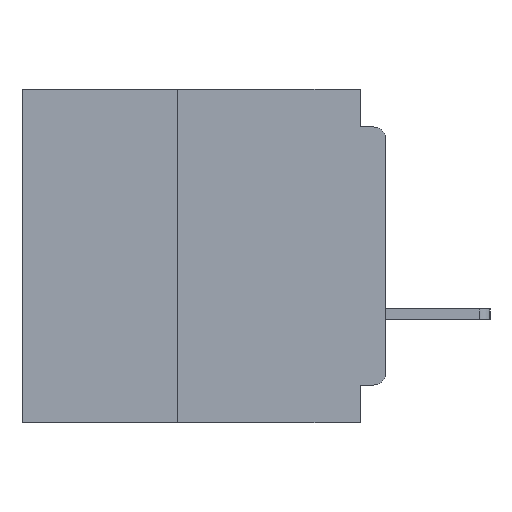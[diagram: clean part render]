
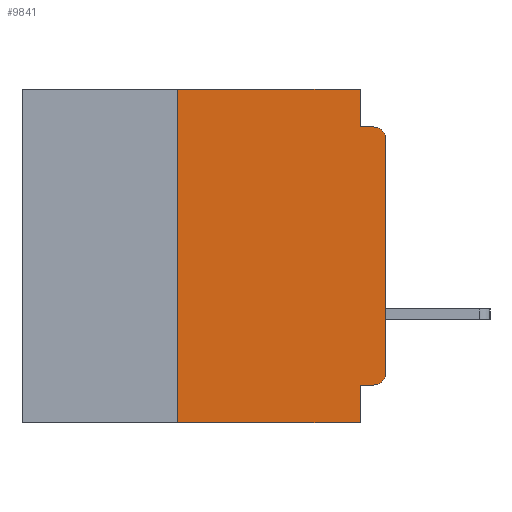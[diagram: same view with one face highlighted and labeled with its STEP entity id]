
A CAD part, left-side view. The second image highlights one B-rep face of the part: STEP entity #9841.
In plain terms, the highlighted planar face has unit normal (-1, 0, 0).
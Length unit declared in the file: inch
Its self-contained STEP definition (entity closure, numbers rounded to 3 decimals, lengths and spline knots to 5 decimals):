
#498 = DIRECTION ( 'NONE',  ( 0., 0., -1. ) ) ;
#1784 = ORIENTED_EDGE ( 'NONE', *, *, #11485, .F. ) ;
#2168 = VECTOR ( 'NONE', #498, 39.37008 ) ;
#2342 = CARTESIAN_POINT ( 'NONE',  ( 0., 0.015, -0.34 ) ) ;
#2679 = CARTESIAN_POINT ( 'NONE',  ( 0., 0.031, 0. ) ) ;
#3452 = DIRECTION ( 'NONE',  ( 0., 0., -1. ) ) ;
#3649 = VECTOR ( 'NONE', #39063, 39.37008 ) ;
#3735 = ORIENTED_EDGE ( 'NONE', *, *, #31207, .T. ) ;
#4716 = DIRECTION ( 'NONE',  ( 0., 1., 0. ) ) ;
#5376 = DIRECTION ( 'NONE',  ( 0., 0., -1. ) ) ;
#5522 = CARTESIAN_POINT ( 'NONE',  ( 0., 0.437, 0. ) ) ;
#5532 = ORIENTED_EDGE ( 'NONE', *, *, #30784, .F. ) ;
#6460 = CARTESIAN_POINT ( 'NONE',  ( 0., 0.015, -0.06 ) ) ;
#6625 = AXIS2_PLACEMENT_3D ( 'NONE', #36912, #30964, #12550 ) ;
#7066 = LINE ( 'NONE', #27614, #14084 ) ;
#7103 = VECTOR ( 'NONE', #31562, 39.37008 ) ;
#7303 = VERTEX_POINT ( 'NONE', #2679 ) ;
#7372 = EDGE_CURVE ( 'NONE', #10352, #23011, #22905, .T. ) ;
#8560 = CARTESIAN_POINT ( 'NONE',  ( 0., 0.25, -0.4 ) ) ;
#8852 = VECTOR ( 'NONE', #4716, 39.37008 ) ;
#9121 = CARTESIAN_POINT ( 'NONE',  ( 0., 0.015, -0.355 ) ) ;
#9322 = AXIS2_PLACEMENT_3D ( 'NONE', #6460, #27766, #9464 ) ;
#9464 = DIRECTION ( 'NONE',  ( 0., 0., -1. ) ) ;
#9841 = ADVANCED_FACE ( 'NONE', ( #22659 ), #27706, .F. ) ;
#9963 = EDGE_CURVE ( 'NONE', #17622, #19025, #16891, .T. ) ;
#10143 = CARTESIAN_POINT ( 'NONE',  ( 0., 0., -0.045 ) ) ;
#10352 = VERTEX_POINT ( 'NONE', #30657 ) ;
#10686 = LINE ( 'NONE', #5522, #3649 ) ;
#11402 = VECTOR ( 'NONE', #35958, 39.37008 ) ;
#11476 = CARTESIAN_POINT ( 'NONE',  ( 0., 0., 0. ) ) ;
#11485 = EDGE_CURVE ( 'NONE', #21725, #7303, #10686, .T. ) ;
#12081 = ORIENTED_EDGE ( 'NONE', *, *, #13093, .T. ) ;
#12195 = DIRECTION ( 'NONE',  ( 0., -1., 0. ) ) ;
#12343 = CARTESIAN_POINT ( 'NONE',  ( 0., 0.031, -0.4 ) ) ;
#12550 = DIRECTION ( 'NONE',  ( 0., 0., -1. ) ) ;
#13093 = EDGE_CURVE ( 'NONE', #17622, #28622, #23886, .T. ) ;
#14084 = VECTOR ( 'NONE', #12195, 39.37008 ) ;
#16891 = LINE ( 'NONE', #32132, #8852 ) ;
#17622 = VERTEX_POINT ( 'NONE', #9121 ) ;
#18445 = ORIENTED_EDGE ( 'NONE', *, *, #36639, .T. ) ;
#18554 = CARTESIAN_POINT ( 'NONE',  ( 0., 0.031, 0. ) ) ;
#19025 = VERTEX_POINT ( 'NONE', #19758 ) ;
#19479 = LINE ( 'NONE', #11476, #11402 ) ;
#19758 = CARTESIAN_POINT ( 'NONE',  ( 0., 0.031, -0.355 ) ) ;
#21395 = EDGE_CURVE ( 'NONE', #23508, #21725, #31826, .T. ) ;
#21725 = VERTEX_POINT ( 'NONE', #36845 ) ;
#22067 = ORIENTED_EDGE ( 'NONE', *, *, #24226, .F. ) ;
#22079 = ORIENTED_EDGE ( 'NONE', *, *, #9963, .F. ) ;
#22505 = AXIS2_PLACEMENT_3D ( 'NONE', #2342, #23511, #5376 ) ;
#22659 = FACE_OUTER_BOUND ( 'NONE', #28017, .T. ) ;
#22905 = CIRCLE ( 'NONE', #9322, 0.015 ) ;
#23011 = VERTEX_POINT ( 'NONE', #33696 ) ;
#23231 = VERTEX_POINT ( 'NONE', #28603 ) ;
#23508 = VERTEX_POINT ( 'NONE', #8560 ) ;
#23511 = DIRECTION ( 'NONE',  ( -1., 0., 0. ) ) ;
#23631 = VECTOR ( 'NONE', #35015, 39.37008 ) ;
#23686 = EDGE_CURVE ( 'NONE', #19025, #23231, #26373, .T. ) ;
#23886 = CIRCLE ( 'NONE', #22505, 0.015 ) ;
#24226 = EDGE_CURVE ( 'NONE', #7303, #28901, #35487, .T. ) ;
#25388 = VECTOR ( 'NONE', #3452, 39.37008 ) ;
#25873 = ORIENTED_EDGE ( 'NONE', *, *, #23686, .F. ) ;
#26373 = LINE ( 'NONE', #12343, #25388 ) ;
#27614 = CARTESIAN_POINT ( 'NONE',  ( 0., 0.437, -0.4 ) ) ;
#27706 = PLANE ( 'NONE',  #6625 ) ;
#27766 = DIRECTION ( 'NONE',  ( -1., 0., 0. ) ) ;
#28017 = EDGE_LOOP ( 'NONE', ( #18445, #36477, #5532, #22067, #1784, #31805, #3735, #25873, #22079, #12081 ) ) ;
#28572 = CARTESIAN_POINT ( 'NONE',  ( 0., 0.031, -0.045 ) ) ;
#28603 = CARTESIAN_POINT ( 'NONE',  ( 0., 0.031, -0.4 ) ) ;
#28622 = VERTEX_POINT ( 'NONE', #33280 ) ;
#28901 = VERTEX_POINT ( 'NONE', #28572 ) ;
#30657 = CARTESIAN_POINT ( 'NONE',  ( 0., 0., -0.06 ) ) ;
#30784 = EDGE_CURVE ( 'NONE', #28901, #23011, #31473, .T. ) ;
#30964 = DIRECTION ( 'NONE',  ( 1., 0., 0. ) ) ;
#31207 = EDGE_CURVE ( 'NONE', #23508, #23231, #7066, .T. ) ;
#31473 = LINE ( 'NONE', #10143, #7103 ) ;
#31562 = DIRECTION ( 'NONE',  ( 0., -1., 0. ) ) ;
#31805 = ORIENTED_EDGE ( 'NONE', *, *, #21395, .F. ) ;
#31826 = LINE ( 'NONE', #31960, #23631 ) ;
#31960 = CARTESIAN_POINT ( 'NONE',  ( 0., 0.25, -0.4 ) ) ;
#32132 = CARTESIAN_POINT ( 'NONE',  ( 0., 0., -0.355 ) ) ;
#33280 = CARTESIAN_POINT ( 'NONE',  ( 0., 0., -0.34 ) ) ;
#33696 = CARTESIAN_POINT ( 'NONE',  ( 0., 0.015, -0.045 ) ) ;
#35015 = DIRECTION ( 'NONE',  ( 0., 0., 1. ) ) ;
#35487 = LINE ( 'NONE', #18554, #2168 ) ;
#35958 = DIRECTION ( 'NONE',  ( 0., 0., 1. ) ) ;
#36477 = ORIENTED_EDGE ( 'NONE', *, *, #7372, .T. ) ;
#36639 = EDGE_CURVE ( 'NONE', #28622, #10352, #19479, .T. ) ;
#36845 = CARTESIAN_POINT ( 'NONE',  ( 0., 0.25, 0. ) ) ;
#36912 = CARTESIAN_POINT ( 'NONE',  ( 0., 0.437, 0. ) ) ;
#39063 = DIRECTION ( 'NONE',  ( 0., -1., 0. ) ) ;
